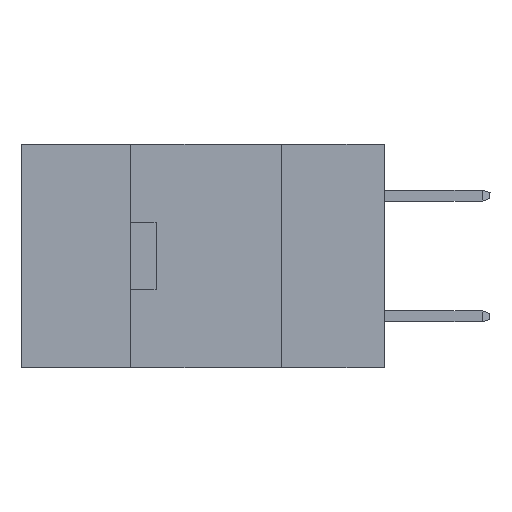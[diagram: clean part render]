
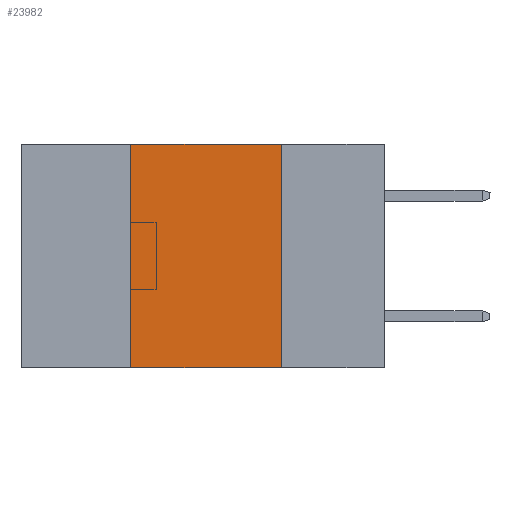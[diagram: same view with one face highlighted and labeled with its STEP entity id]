
A CAD part, left-side view. The second image highlights one B-rep face of the part: STEP entity #23982.
In plain terms, the highlighted planar face has unit normal (-1, 0, 0).
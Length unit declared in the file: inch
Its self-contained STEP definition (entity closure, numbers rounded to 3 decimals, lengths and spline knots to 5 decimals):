
#217 = LINE ( 'NONE', #19176, #1629 ) ;
#616 = VECTOR ( 'NONE', #21290, 39.37008 ) ;
#773 = CARTESIAN_POINT ( 'NONE',  ( 0., 0.6, 0. ) ) ;
#1027 = AXIS2_PLACEMENT_3D ( 'NONE', #773, #5249, #20379 ) ;
#1116 = ORIENTED_EDGE ( 'NONE', *, *, #19233, .F. ) ;
#1238 = ORIENTED_EDGE ( 'NONE', *, *, #22972, .T. ) ;
#1629 = VECTOR ( 'NONE', #6186, 39.37008 ) ;
#1953 = VERTEX_POINT ( 'NONE', #11226 ) ;
#3008 = PLANE ( 'NONE',  #1027 ) ;
#4003 = CARTESIAN_POINT ( 'NONE',  ( 0., 0.6, 0. ) ) ;
#5249 = DIRECTION ( 'NONE',  ( 1., 0., 0. ) ) ;
#6186 = DIRECTION ( 'NONE',  ( 0., 0., 1. ) ) ;
#6524 = LINE ( 'NONE', #4003, #616 ) ;
#6764 = CARTESIAN_POINT ( 'NONE',  ( 0., 0.42, -0.37 ) ) ;
#8884 = VERTEX_POINT ( 'NONE', #27109 ) ;
#9559 = DIRECTION ( 'NONE',  ( 0., 0., -1. ) ) ;
#9800 = VERTEX_POINT ( 'NONE', #17286 ) ;
#11226 = CARTESIAN_POINT ( 'NONE',  ( 0., 0.17, 0. ) ) ;
#13963 = EDGE_CURVE ( 'NONE', #9800, #1953, #6524, .T. ) ;
#14126 = VERTEX_POINT ( 'NONE', #6764 ) ;
#15674 = ORIENTED_EDGE ( 'NONE', *, *, #27542, .F. ) ;
#16038 = EDGE_LOOP ( 'NONE', ( #1116, #17064, #15674, #1238 ) ) ;
#17064 = ORIENTED_EDGE ( 'NONE', *, *, #13963, .F. ) ;
#17286 = CARTESIAN_POINT ( 'NONE',  ( 0., 0.42, 0. ) ) ;
#17403 = LINE ( 'NONE', #21531, #27905 ) ;
#19031 = VECTOR ( 'NONE', #9559, 39.37008 ) ;
#19176 = CARTESIAN_POINT ( 'NONE',  ( 0., 0.42, -0.37 ) ) ;
#19233 = EDGE_CURVE ( 'NONE', #1953, #8884, #24593, .T. ) ;
#20276 = CARTESIAN_POINT ( 'NONE',  ( 0., 0.17, -0.37 ) ) ;
#20379 = DIRECTION ( 'NONE',  ( 0., 0., -1. ) ) ;
#21290 = DIRECTION ( 'NONE',  ( 0., -1., 0. ) ) ;
#21531 = CARTESIAN_POINT ( 'NONE',  ( 0., 0.6, -0.37 ) ) ;
#22972 = EDGE_CURVE ( 'NONE', #14126, #8884, #17403, .T. ) ;
#23629 = DIRECTION ( 'NONE',  ( 0., -1., 0. ) ) ;
#23982 = ADVANCED_FACE ( 'NONE', ( #24559 ), #3008, .F. ) ;
#24559 = FACE_OUTER_BOUND ( 'NONE', #16038, .T. ) ;
#24593 = LINE ( 'NONE', #20276, #19031 ) ;
#27109 = CARTESIAN_POINT ( 'NONE',  ( 0., 0.17, -0.37 ) ) ;
#27542 = EDGE_CURVE ( 'NONE', #14126, #9800, #217, .T. ) ;
#27905 = VECTOR ( 'NONE', #23629, 39.37008 ) ;
